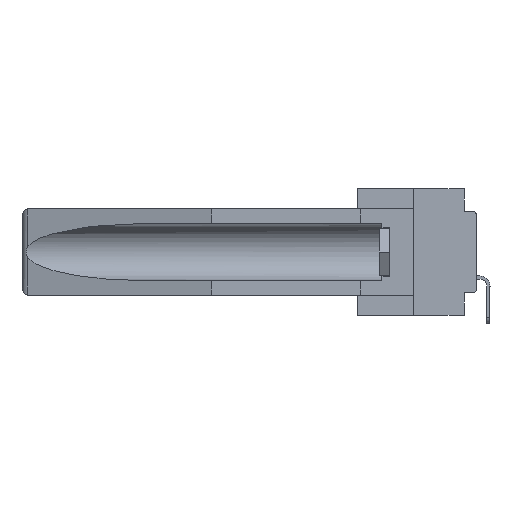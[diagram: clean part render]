
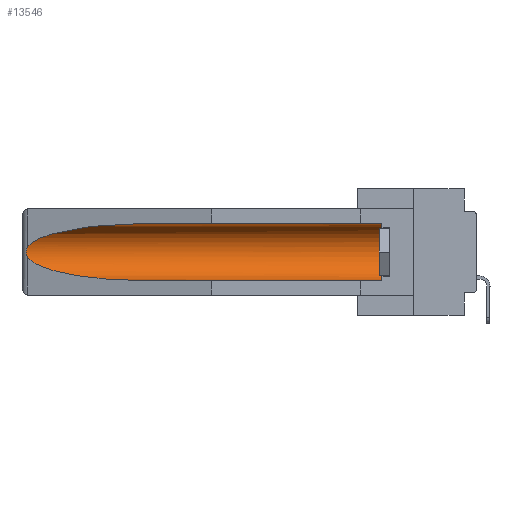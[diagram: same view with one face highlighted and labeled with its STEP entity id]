
A CAD part, left-side view. The second image highlights one B-rep face of the part: STEP entity #13546.
In plain terms, the highlighted cylindrical face has radius 2.857 mm (diameter 5.715 mm), a partial arc.
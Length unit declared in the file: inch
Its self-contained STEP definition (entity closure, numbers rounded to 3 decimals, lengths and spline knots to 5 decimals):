
#466 = CARTESIAN_POINT ( 'NONE',  ( 0.26537, 1.52718, -0.14972 ) ) ;
#544 = CARTESIAN_POINT ( 'NONE',  ( 0.26597, 1.52961, -0.15275 ) ) ;
#1689 = CARTESIAN_POINT ( 'NONE',  ( 0.155, -0.30754, -0.1715 ) ) ;
#2208 = FACE_OUTER_BOUND ( 'NONE', #10056, .T. ) ;
#2246 = CYLINDRICAL_SURFACE ( 'NONE', #17385, 0.1125 ) ;
#2670 = CARTESIAN_POINT ( 'NONE',  ( 0.155, 0.126, -0.059 ) ) ;
#2793 =( BOUNDED_CURVE ( )  B_SPLINE_CURVE ( 3, ( #7959, #24004, #31771, #23552 ),
 .UNSPECIFIED., .F., .F. ) 
 B_SPLINE_CURVE_WITH_KNOTS ( ( 4, 4 ),
 ( 0.1948, 1.5708 ),
 .UNSPECIFIED. ) 
 CURVE ( )  GEOMETRIC_REPRESENTATION_ITEM ( )  RATIONAL_B_SPLINE_CURVE ( ( 1., 0.848, 0.848, 1. ) ) 
 REPRESENTATION_ITEM ( '' )  );
#2799 = CARTESIAN_POINT ( 'NONE',  ( 0.21114, 1.30732, -0.059 ) ) ;
#4637 = EDGE_CURVE ( 'NONE', #31270, #28307, #10999, .T. ) ;
#4676 = DIRECTION ( 'NONE',  ( 0., 0., 1. ) ) ;
#5540 = EDGE_CURVE ( 'NONE', #28307, #17166, #2793, .T. ) ;
#6473 = VERTEX_POINT ( 'NONE', #11297 ) ;
#7194 = DIRECTION ( 'NONE',  ( 0., 1., 0. ) ) ;
#7209 = VERTEX_POINT ( 'NONE', #2670 ) ;
#7273 = DIRECTION ( 'NONE',  ( 0., 0., 1. ) ) ;
#7959 = CARTESIAN_POINT ( 'NONE',  ( 0.26537, 1.52718, -0.19328 ) ) ;
#7986 = VECTOR ( 'NONE', #22145, 39.37008 ) ;
#8063 = CARTESIAN_POINT ( 'NONE',  ( 0.25451, 1.48313, -0.09465 ) ) ;
#8165 = ORIENTED_EDGE ( 'NONE', *, *, #9562, .T. ) ;
#8361 = CARTESIAN_POINT ( 'NONE',  ( 0.26597, 1.5296, -0.19026 ) ) ;
#9562 = EDGE_CURVE ( 'NONE', #6473, #7209, #25637, .T. ) ;
#10056 = EDGE_LOOP ( 'NONE', ( #20772, #21328, #29204, #14153, #8165, #25302 ) ) ;
#10353 = CARTESIAN_POINT ( 'NONE',  ( 0.155, 1.07973, -0.059 ) ) ;
#10999 = B_SPLINE_CURVE_WITH_KNOTS ( 'NONE', 3,
 ( #24084, #544, #18797, #29621, #13803, #32279, #16230, #32391, #8361, #21765 ),
 .UNSPECIFIED., .F., .F.,
 ( 4, 2, 2, 2, 4 ),
 ( 0., 0.00029, 0.00058, 0.00087, 0.00117 ),
 .UNSPECIFIED. ) ;
#11297 = CARTESIAN_POINT ( 'NONE',  ( 0.155, 0.126, -0.284 ) ) ;
#12931 = EDGE_CURVE ( 'NONE', #7209, #30465, #31167, .T. ) ;
#13546 = ADVANCED_FACE ( 'NONE', ( #2208 ), #2246, .F. ) ;
#13803 = CARTESIAN_POINT ( 'NONE',  ( 0.2675, 1.53308, -0.16763 ) ) ;
#14153 = ORIENTED_EDGE ( 'NONE', *, *, #18375, .F. ) ;
#16230 = CARTESIAN_POINT ( 'NONE',  ( 0.2673, 1.53269, -0.17917 ) ) ;
#16382 = CARTESIAN_POINT ( 'NONE',  ( 0.155, 1.07973, -0.059 ) ) ;
#16398 = CARTESIAN_POINT ( 'NONE',  ( 0.26537, 1.52718, -0.14972 ) ) ;
#17166 = VERTEX_POINT ( 'NONE', #20863 ) ;
#17385 = AXIS2_PLACEMENT_3D ( 'NONE', #1689, #7194, #4676 ) ;
#18375 = EDGE_CURVE ( 'NONE', #6473, #17166, #25616, .T. ) ;
#18797 = CARTESIAN_POINT ( 'NONE',  ( 0.26654, 1.53092, -0.15636 ) ) ;
#20094 = CARTESIAN_POINT ( 'NONE',  ( 0.26537, 1.52718, -0.19328 ) ) ;
#20772 = ORIENTED_EDGE ( 'NONE', *, *, #27941, .T. ) ;
#20863 = CARTESIAN_POINT ( 'NONE',  ( 0.155, 1.07973, -0.284 ) ) ;
#21087 = VECTOR ( 'NONE', #29077, 39.37008 ) ;
#21328 = ORIENTED_EDGE ( 'NONE', *, *, #4637, .T. ) ;
#21765 = CARTESIAN_POINT ( 'NONE',  ( 0.26537, 1.52718, -0.19328 ) ) ;
#22145 = DIRECTION ( 'NONE',  ( 0., 1., 0. ) ) ;
#23093 = CARTESIAN_POINT ( 'NONE',  ( 0.155, 0.126, -0.1715 ) ) ;
#23552 = CARTESIAN_POINT ( 'NONE',  ( 0.155, 1.07973, -0.284 ) ) ;
#24004 = CARTESIAN_POINT ( 'NONE',  ( 0.25451, 1.48313, -0.24835 ) ) ;
#24084 = CARTESIAN_POINT ( 'NONE',  ( 0.26537, 1.52718, -0.14972 ) ) ;
#25246 = AXIS2_PLACEMENT_3D ( 'NONE', #23093, #25878, #7273 ) ;
#25302 = ORIENTED_EDGE ( 'NONE', *, *, #12931, .T. ) ;
#25616 = LINE ( 'NONE', #31727, #21087 ) ;
#25637 = CIRCLE ( 'NONE', #25246, 0.1125 ) ;
#25878 = DIRECTION ( 'NONE',  ( 0., -1., 0. ) ) ;
#27323 = CARTESIAN_POINT ( 'NONE',  ( 0.155, -0.30754, -0.059 ) ) ;
#27941 = EDGE_CURVE ( 'NONE', #30465, #31270, #34083, .T. ) ;
#28307 = VERTEX_POINT ( 'NONE', #20094 ) ;
#29077 = DIRECTION ( 'NONE',  ( 0., 1., 0. ) ) ;
#29204 = ORIENTED_EDGE ( 'NONE', *, *, #5540, .T. ) ;
#29621 = CARTESIAN_POINT ( 'NONE',  ( 0.2673, 1.5327, -0.16383 ) ) ;
#30465 = VERTEX_POINT ( 'NONE', #10353 ) ;
#31167 = LINE ( 'NONE', #27323, #7986 ) ;
#31270 = VERTEX_POINT ( 'NONE', #16398 ) ;
#31727 = CARTESIAN_POINT ( 'NONE',  ( 0.155, -0.30754, -0.284 ) ) ;
#31771 = CARTESIAN_POINT ( 'NONE',  ( 0.21114, 1.30732, -0.284 ) ) ;
#32279 = CARTESIAN_POINT ( 'NONE',  ( 0.2675, 1.53308, -0.17534 ) ) ;
#32391 = CARTESIAN_POINT ( 'NONE',  ( 0.26655, 1.53094, -0.18657 ) ) ;
#34083 =( BOUNDED_CURVE ( )  B_SPLINE_CURVE ( 3, ( #16382, #2799, #8063, #466 ),
 .UNSPECIFIED., .F., .F. ) 
 B_SPLINE_CURVE_WITH_KNOTS ( ( 4, 4 ),
 ( 4.71239, 6.08839 ),
 .UNSPECIFIED. ) 
 CURVE ( )  GEOMETRIC_REPRESENTATION_ITEM ( )  RATIONAL_B_SPLINE_CURVE ( ( 1., 0.848, 0.848, 1. ) ) 
 REPRESENTATION_ITEM ( '' )  );
